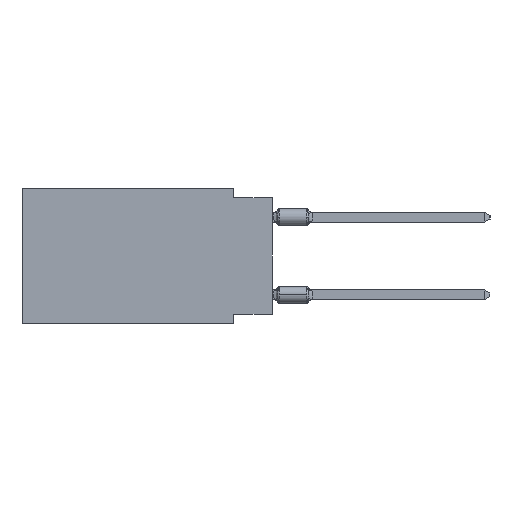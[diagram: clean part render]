
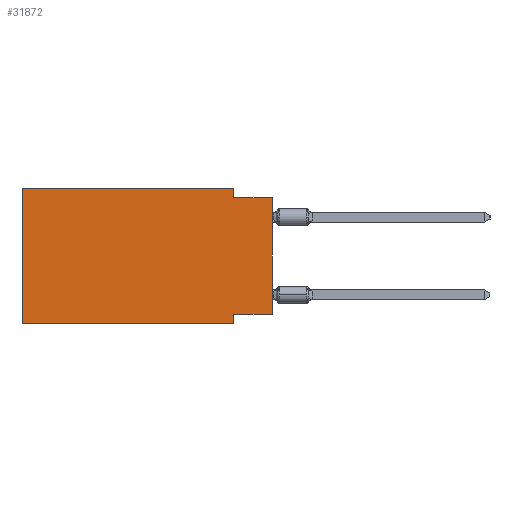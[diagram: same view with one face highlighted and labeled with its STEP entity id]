
A CAD part, left-side view. The second image highlights one B-rep face of the part: STEP entity #31872.
In plain terms, the highlighted planar face has unit normal (-1, 0, 0).
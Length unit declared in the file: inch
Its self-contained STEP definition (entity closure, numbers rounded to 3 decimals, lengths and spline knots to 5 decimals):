
#1018 = VECTOR ( 'NONE', #32170, 39.37008 ) ;
#2329 = DIRECTION ( 'NONE',  ( 0., 1., 0. ) ) ;
#3799 = LINE ( 'NONE', #22760, #41893 ) ;
#4818 = VERTEX_POINT ( 'NONE', #25721 ) ;
#4907 = EDGE_CURVE ( 'NONE', #11419, #23622, #3799, .T. ) ;
#5399 = LINE ( 'NONE', #14382, #37482 ) ;
#5501 = CARTESIAN_POINT ( 'NONE',  ( 0., 0., -0.325 ) ) ;
#5751 = VERTEX_POINT ( 'NONE', #19819 ) ;
#6133 = VERTEX_POINT ( 'NONE', #18214 ) ;
#7123 = LINE ( 'NONE', #20107, #11194 ) ;
#7282 = CARTESIAN_POINT ( 'NONE',  ( 0., 0.645, 0. ) ) ;
#7294 = EDGE_CURVE ( 'NONE', #10034, #4818, #15730, .T. ) ;
#7728 = DIRECTION ( 'NONE',  ( 0., 0., -1. ) ) ;
#8006 = CARTESIAN_POINT ( 'NONE',  ( 0., 0., 0. ) ) ;
#10034 = VERTEX_POINT ( 'NONE', #21050 ) ;
#10851 = EDGE_CURVE ( 'NONE', #23622, #14189, #7123, .T. ) ;
#11064 = EDGE_CURVE ( 'NONE', #4818, #5751, #41750, .T. ) ;
#11194 = VECTOR ( 'NONE', #33060, 39.37008 ) ;
#11419 = VERTEX_POINT ( 'NONE', #13563 ) ;
#12459 = VECTOR ( 'NONE', #39688, 39.37008 ) ;
#12845 = DIRECTION ( 'NONE',  ( 0., 0., -1. ) ) ;
#13563 = CARTESIAN_POINT ( 'NONE',  ( 0., 0.645, -0.35 ) ) ;
#14189 = VERTEX_POINT ( 'NONE', #30563 ) ;
#14382 = CARTESIAN_POINT ( 'NONE',  ( 0., 0., -0.025 ) ) ;
#14741 = EDGE_CURVE ( 'NONE', #14189, #6133, #35372, .T. ) ;
#14804 = VECTOR ( 'NONE', #12845, 39.37008 ) ;
#15587 = CARTESIAN_POINT ( 'NONE',  ( 0., 0., -0.025 ) ) ;
#15730 = LINE ( 'NONE', #5501, #36851 ) ;
#15854 = VECTOR ( 'NONE', #28144, 39.37008 ) ;
#16241 = ORIENTED_EDGE ( 'NONE', *, *, #10851, .F. ) ;
#16259 = ORIENTED_EDGE ( 'NONE', *, *, #7294, .F. ) ;
#16783 = DIRECTION ( 'NONE',  ( 0., 0., 1. ) ) ;
#17670 = ORIENTED_EDGE ( 'NONE', *, *, #11064, .F. ) ;
#17794 = LINE ( 'NONE', #8006, #12459 ) ;
#18214 = CARTESIAN_POINT ( 'NONE',  ( 0., 0.1, -0.025 ) ) ;
#19016 = CARTESIAN_POINT ( 'NONE',  ( 0., 0.1, -0.35 ) ) ;
#19307 = FACE_OUTER_BOUND ( 'NONE', #23574, .T. ) ;
#19819 = CARTESIAN_POINT ( 'NONE',  ( 0., 0.1, -0.35 ) ) ;
#20107 = CARTESIAN_POINT ( 'NONE',  ( 0., 0.645, 0. ) ) ;
#21050 = CARTESIAN_POINT ( 'NONE',  ( 0., 0., -0.325 ) ) ;
#21996 = CARTESIAN_POINT ( 'NONE',  ( 0., 0.1, 0. ) ) ;
#22760 = CARTESIAN_POINT ( 'NONE',  ( 0., 0.645, 0. ) ) ;
#22937 = DIRECTION ( 'NONE',  ( 1., 0., 0. ) ) ;
#23574 = EDGE_LOOP ( 'NONE', ( #23994, #29690, #28649, #16241, #26039, #33362, #17670, #16259 ) ) ;
#23622 = VERTEX_POINT ( 'NONE', #7282 ) ;
#23994 = ORIENTED_EDGE ( 'NONE', *, *, #39782, .T. ) ;
#25165 = CARTESIAN_POINT ( 'NONE',  ( 0., 0.645, -0.35 ) ) ;
#25721 = CARTESIAN_POINT ( 'NONE',  ( 0., 0.1, -0.325 ) ) ;
#26039 = ORIENTED_EDGE ( 'NONE', *, *, #4907, .F. ) ;
#26824 = EDGE_CURVE ( 'NONE', #11419, #5751, #31539, .T. ) ;
#28144 = DIRECTION ( 'NONE',  ( 0., -1., 0. ) ) ;
#28649 = ORIENTED_EDGE ( 'NONE', *, *, #14741, .F. ) ;
#29267 = PLANE ( 'NONE',  #35051 ) ;
#29690 = ORIENTED_EDGE ( 'NONE', *, *, #33819, .F. ) ;
#30563 = CARTESIAN_POINT ( 'NONE',  ( 0., 0.1, 0. ) ) ;
#31539 = LINE ( 'NONE', #25165, #15854 ) ;
#31872 = ADVANCED_FACE ( 'NONE', ( #19307 ), #29267, .F. ) ;
#32170 = DIRECTION ( 'NONE',  ( 0., 0., -1. ) ) ;
#33060 = DIRECTION ( 'NONE',  ( 0., -1., 0. ) ) ;
#33362 = ORIENTED_EDGE ( 'NONE', *, *, #26824, .T. ) ;
#33819 = EDGE_CURVE ( 'NONE', #6133, #40616, #5399, .T. ) ;
#35051 = AXIS2_PLACEMENT_3D ( 'NONE', #40053, #22937, #7728 ) ;
#35372 = LINE ( 'NONE', #21996, #14804 ) ;
#36851 = VECTOR ( 'NONE', #2329, 39.37008 ) ;
#37329 = DIRECTION ( 'NONE',  ( 0., -1., 0. ) ) ;
#37482 = VECTOR ( 'NONE', #37329, 39.37008 ) ;
#39688 = DIRECTION ( 'NONE',  ( 0., 0., 1. ) ) ;
#39782 = EDGE_CURVE ( 'NONE', #10034, #40616, #17794, .T. ) ;
#40053 = CARTESIAN_POINT ( 'NONE',  ( 0., 0.645, 0. ) ) ;
#40616 = VERTEX_POINT ( 'NONE', #15587 ) ;
#41750 = LINE ( 'NONE', #19016, #1018 ) ;
#41893 = VECTOR ( 'NONE', #16783, 39.37008 ) ;
